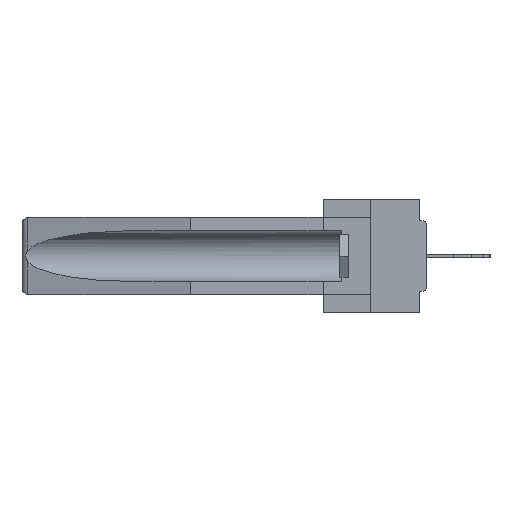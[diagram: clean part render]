
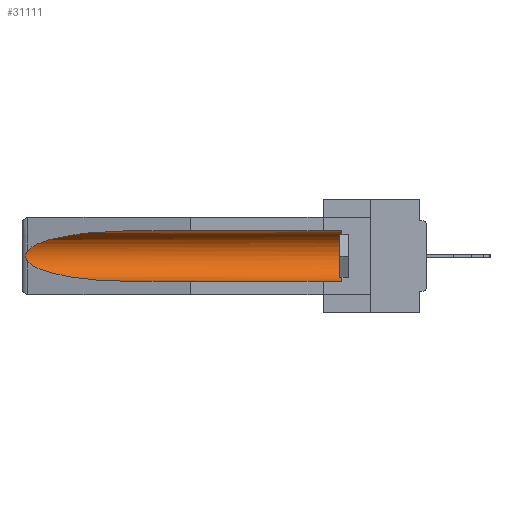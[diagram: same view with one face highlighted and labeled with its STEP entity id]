
A CAD part, left-side view. The second image highlights one B-rep face of the part: STEP entity #31111.
In plain terms, the highlighted cylindrical face has radius 2.857 mm (diameter 5.715 mm), a partial arc.
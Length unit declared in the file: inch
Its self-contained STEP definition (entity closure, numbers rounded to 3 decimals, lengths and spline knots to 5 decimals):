
#6 = EDGE_CURVE ( 'NONE', #14723, #2886, #31071, .T. ) ;
#362 = ORIENTED_EDGE ( 'NONE', *, *, #9070, .T. ) ;
#822 = VERTEX_POINT ( 'NONE', #15905 ) ;
#1792 = CARTESIAN_POINT ( 'NONE',  ( 0.26537, 1.52718, -0.19328 ) ) ;
#2364 = VERTEX_POINT ( 'NONE', #7890 ) ;
#2886 = VERTEX_POINT ( 'NONE', #6630 ) ;
#3351 = CARTESIAN_POINT ( 'NONE',  ( 0.155, -0.30754, -0.059 ) ) ;
#4242 = CARTESIAN_POINT ( 'NONE',  ( 0.26537, 1.52718, -0.19328 ) ) ;
#5216 = ORIENTED_EDGE ( 'NONE', *, *, #6, .T. ) ;
#5321 = EDGE_LOOP ( 'NONE', ( #30585, #16857, #5216, #36475, #362, #10205 ) ) ;
#6271 = CARTESIAN_POINT ( 'NONE',  ( 0.2673, 1.53269, -0.17917 ) ) ;
#6459 = CARTESIAN_POINT ( 'NONE',  ( 0.2673, 1.5327, -0.16383 ) ) ;
#6630 = CARTESIAN_POINT ( 'NONE',  ( 0.155, 1.07973, -0.284 ) ) ;
#6803 = CARTESIAN_POINT ( 'NONE',  ( 0.155, 1.07973, -0.059 ) ) ;
#7890 = CARTESIAN_POINT ( 'NONE',  ( 0.155, 0.126, -0.059 ) ) ;
#8965 = LINE ( 'NONE', #3351, #13528 ) ;
#9070 = EDGE_CURVE ( 'NONE', #28904, #2364, #11503, .T. ) ;
#9249 = CARTESIAN_POINT ( 'NONE',  ( 0.21114, 1.30732, -0.059 ) ) ;
#9638 = CARTESIAN_POINT ( 'NONE',  ( 0.26537, 1.52718, -0.19328 ) ) ;
#9888 = VERTEX_POINT ( 'NONE', #6803 ) ;
#10205 = ORIENTED_EDGE ( 'NONE', *, *, #11839, .T. ) ;
#11503 = CIRCLE ( 'NONE', #32403, 0.1125 ) ;
#11839 = EDGE_CURVE ( 'NONE', #2364, #9888, #8965, .T. ) ;
#11850 = CARTESIAN_POINT ( 'NONE',  ( 0.26537, 1.52718, -0.14972 ) ) ;
#12311 = DIRECTION ( 'NONE',  ( 0., 1., 0. ) ) ;
#12365 = DIRECTION ( 'NONE',  ( 0., 0., 1. ) ) ;
#13138 = CARTESIAN_POINT ( 'NONE',  ( 0.26654, 1.53092, -0.15636 ) ) ;
#13528 = VECTOR ( 'NONE', #14755, 39.37008 ) ;
#14723 = VERTEX_POINT ( 'NONE', #1792 ) ;
#14755 = DIRECTION ( 'NONE',  ( 0., 1., 0. ) ) ;
#14863 = CARTESIAN_POINT ( 'NONE',  ( 0.26655, 1.53094, -0.18657 ) ) ;
#15124 = CARTESIAN_POINT ( 'NONE',  ( 0.155, -0.30754, -0.1715 ) ) ;
#15546 = B_SPLINE_CURVE_WITH_KNOTS ( 'NONE', 3,
 ( #18759, #34883, #13138, #6459, #35955, #29268, #6271, #14863, #17864, #9638 ),
 .UNSPECIFIED., .F., .F.,
 ( 4, 2, 2, 2, 4 ),
 ( 0., 0.00029, 0.00058, 0.00087, 0.00117 ),
 .UNSPECIFIED. ) ;
#15905 = CARTESIAN_POINT ( 'NONE',  ( 0.26537, 1.52718, -0.14972 ) ) ;
#16857 = ORIENTED_EDGE ( 'NONE', *, *, #24912, .T. ) ;
#17864 = CARTESIAN_POINT ( 'NONE',  ( 0.26597, 1.5296, -0.19026 ) ) ;
#18306 = CARTESIAN_POINT ( 'NONE',  ( 0.155, -0.30754, -0.284 ) ) ;
#18759 = CARTESIAN_POINT ( 'NONE',  ( 0.26537, 1.52718, -0.14972 ) ) ;
#20652 = CARTESIAN_POINT ( 'NONE',  ( 0.155, 1.07973, -0.059 ) ) ;
#22902 = CARTESIAN_POINT ( 'NONE',  ( 0.25451, 1.48313, -0.09465 ) ) ;
#23194 = DIRECTION ( 'NONE',  ( 0., 1., 0. ) ) ;
#23904 = CARTESIAN_POINT ( 'NONE',  ( 0.21114, 1.30732, -0.284 ) ) ;
#24912 = EDGE_CURVE ( 'NONE', #822, #14723, #15546, .T. ) ;
#25274 = EDGE_CURVE ( 'NONE', #9888, #822, #27030, .T. ) ;
#26245 = EDGE_CURVE ( 'NONE', #28904, #2886, #34953, .T. ) ;
#27030 =( BOUNDED_CURVE ( )  B_SPLINE_CURVE ( 3, ( #20652, #9249, #22902, #11850 ),
 .UNSPECIFIED., .F., .F. ) 
 B_SPLINE_CURVE_WITH_KNOTS ( ( 4, 4 ),
 ( 4.71239, 6.08839 ),
 .UNSPECIFIED. ) 
 CURVE ( )  GEOMETRIC_REPRESENTATION_ITEM ( )  RATIONAL_B_SPLINE_CURVE ( ( 1., 0.848, 0.848, 1. ) ) 
 REPRESENTATION_ITEM ( '' )  );
#27995 = VECTOR ( 'NONE', #12311, 39.37008 ) ;
#28904 = VERTEX_POINT ( 'NONE', #36827 ) ;
#29268 = CARTESIAN_POINT ( 'NONE',  ( 0.2675, 1.53308, -0.17534 ) ) ;
#29362 = AXIS2_PLACEMENT_3D ( 'NONE', #15124, #23194, #32316 ) ;
#29499 = CARTESIAN_POINT ( 'NONE',  ( 0.25451, 1.48313, -0.24835 ) ) ;
#30585 = ORIENTED_EDGE ( 'NONE', *, *, #25274, .T. ) ;
#31071 =( BOUNDED_CURVE ( )  B_SPLINE_CURVE ( 3, ( #4242, #29499, #23904, #34930 ),
 .UNSPECIFIED., .F., .F. ) 
 B_SPLINE_CURVE_WITH_KNOTS ( ( 4, 4 ),
 ( 0.1948, 1.5708 ),
 .UNSPECIFIED. ) 
 CURVE ( )  GEOMETRIC_REPRESENTATION_ITEM ( )  RATIONAL_B_SPLINE_CURVE ( ( 1., 0.848, 0.848, 1. ) ) 
 REPRESENTATION_ITEM ( '' )  );
#31111 = ADVANCED_FACE ( 'NONE', ( #31601 ), #35146, .F. ) ;
#31601 = FACE_OUTER_BOUND ( 'NONE', #5321, .T. ) ;
#32316 = DIRECTION ( 'NONE',  ( 0., 0., 1. ) ) ;
#32403 = AXIS2_PLACEMENT_3D ( 'NONE', #34626, #35009, #12365 ) ;
#34626 = CARTESIAN_POINT ( 'NONE',  ( 0.155, 0.126, -0.1715 ) ) ;
#34883 = CARTESIAN_POINT ( 'NONE',  ( 0.26597, 1.52961, -0.15275 ) ) ;
#34930 = CARTESIAN_POINT ( 'NONE',  ( 0.155, 1.07973, -0.284 ) ) ;
#34953 = LINE ( 'NONE', #18306, #27995 ) ;
#35009 = DIRECTION ( 'NONE',  ( 0., -1., 0. ) ) ;
#35146 = CYLINDRICAL_SURFACE ( 'NONE', #29362, 0.1125 ) ;
#35955 = CARTESIAN_POINT ( 'NONE',  ( 0.2675, 1.53308, -0.16763 ) ) ;
#36475 = ORIENTED_EDGE ( 'NONE', *, *, #26245, .F. ) ;
#36827 = CARTESIAN_POINT ( 'NONE',  ( 0.155, 0.126, -0.284 ) ) ;
